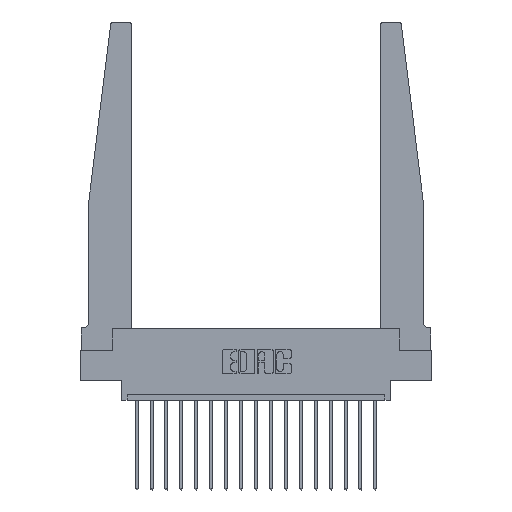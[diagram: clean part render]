
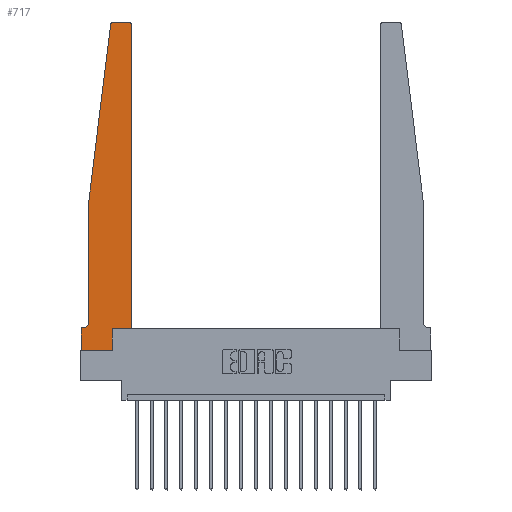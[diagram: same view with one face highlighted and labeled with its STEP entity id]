
A CAD part, top view. The second image highlights one B-rep face of the part: STEP entity #717.
In plain terms, the highlighted planar face has unit normal (0, 0, 1).
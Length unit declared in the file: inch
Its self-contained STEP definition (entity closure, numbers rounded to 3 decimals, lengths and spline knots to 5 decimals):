
#295 = CARTESIAN_POINT ( 'NONE',  ( 0.425, 0.18, 0.37 ) ) ;
#332 = LINE ( 'NONE', #9347, #19190 ) ;
#488 = DIRECTION ( 'NONE',  ( 1., 0., 0. ) ) ;
#708 = CARTESIAN_POINT ( 'NONE',  ( 0.2605, 0.18, 0.37 ) ) ;
#717 = ADVANCED_FACE ( 'NONE', ( #12326 ), #10765, .T. ) ;
#748 = CARTESIAN_POINT ( 'NONE',  ( 0.395, 2.75, 0.37 ) ) ;
#1298 = VERTEX_POINT ( 'NONE', #6722 ) ;
#1452 = EDGE_CURVE ( 'NONE', #1948, #12382, #332, .T. ) ;
#1479 = ORIENTED_EDGE ( 'NONE', *, *, #14520, .T. ) ;
#1593 = VERTEX_POINT ( 'NONE', #708 ) ;
#1856 = CARTESIAN_POINT ( 'NONE',  ( 0., 0.1875, 0.37 ) ) ;
#1948 = VERTEX_POINT ( 'NONE', #12718 ) ;
#2142 = CARTESIAN_POINT ( 'NONE',  ( 0.27653, 2.72, 0.37 ) ) ;
#3500 = CARTESIAN_POINT ( 'NONE',  ( 0., 0., 0.37 ) ) ;
#3539 = EDGE_CURVE ( 'NONE', #6648, #1298, #10495, .T. ) ;
#4411 = DIRECTION ( 'NONE',  ( -1., 0., 0. ) ) ;
#4610 = AXIS2_PLACEMENT_3D ( 'NONE', #1856, #7816, #14106 ) ;
#4920 = DIRECTION ( 'NONE',  ( 0., 1., 0. ) ) ;
#5121 = VECTOR ( 'NONE', #4411, 39.37008 ) ;
#5451 = VERTEX_POINT ( 'NONE', #6592 ) ;
#5759 = EDGE_CURVE ( 'NONE', #8194, #7303, #10696, .T. ) ;
#5933 = LINE ( 'NONE', #10330, #7290 ) ;
#6024 = VERTEX_POINT ( 'NONE', #8414 ) ;
#6096 = CIRCLE ( 'NONE', #14825, 0.05 ) ;
#6125 = DIRECTION ( 'NONE',  ( 1., 0., 0. ) ) ;
#6316 = CARTESIAN_POINT ( 'NONE',  ( 0.065, 1.25, 0.37 ) ) ;
#6592 = CARTESIAN_POINT ( 'NONE',  ( 0.425, 0.18, 0.37 ) ) ;
#6648 = VERTEX_POINT ( 'NONE', #6976 ) ;
#6722 = CARTESIAN_POINT ( 'NONE',  ( 0.24675, 2.72367, 0.37 ) ) ;
#6766 = DIRECTION ( 'NONE',  ( 0., 0., 1. ) ) ;
#6798 = CARTESIAN_POINT ( 'NONE',  ( 0., 0.1875, 0.37 ) ) ;
#6899 = CARTESIAN_POINT ( 'NONE',  ( 0.065, 0.1875, 0.37 ) ) ;
#6976 = CARTESIAN_POINT ( 'NONE',  ( 0.27653, 2.75, 0.37 ) ) ;
#7077 = ORIENTED_EDGE ( 'NONE', *, *, #9701, .T. ) ;
#7096 = ORIENTED_EDGE ( 'NONE', *, *, #13412, .T. ) ;
#7290 = VECTOR ( 'NONE', #7386, 39.37008 ) ;
#7303 = VERTEX_POINT ( 'NONE', #748 ) ;
#7348 = LINE ( 'NONE', #17659, #5121 ) ;
#7386 = DIRECTION ( 'NONE',  ( 1., 0., 0. ) ) ;
#7409 = ORIENTED_EDGE ( 'NONE', *, *, #5759, .T. ) ;
#7816 = DIRECTION ( 'NONE',  ( 0., 0., 1. ) ) ;
#8069 = DIRECTION ( 'NONE',  ( -0.122, -0.992, 0. ) ) ;
#8194 = VERTEX_POINT ( 'NONE', #18931 ) ;
#8267 = EDGE_CURVE ( 'NONE', #1298, #16769, #15222, .T. ) ;
#8414 = CARTESIAN_POINT ( 'NONE',  ( 0.065, 0.2375, 0.37 ) ) ;
#8739 = ORIENTED_EDGE ( 'NONE', *, *, #10263, .T. ) ;
#8806 = EDGE_CURVE ( 'NONE', #12382, #1593, #18109, .T. ) ;
#8812 = AXIS2_PLACEMENT_3D ( 'NONE', #13911, #6766, #488 ) ;
#8829 = DIRECTION ( 'NONE',  ( -1., 0., 0. ) ) ;
#9012 = VERTEX_POINT ( 'NONE', #12609 ) ;
#9017 = DIRECTION ( 'NONE',  ( 1., 0., 0. ) ) ;
#9347 = CARTESIAN_POINT ( 'NONE',  ( 0., 0., 0.37 ) ) ;
#9701 = EDGE_CURVE ( 'NONE', #1593, #5451, #5933, .T. ) ;
#10263 = EDGE_CURVE ( 'NONE', #5451, #8194, #12343, .T. ) ;
#10330 = CARTESIAN_POINT ( 'NONE',  ( 0.425, 0.18, 0.37 ) ) ;
#10352 = VECTOR ( 'NONE', #12438, 39.37008 ) ;
#10495 = CIRCLE ( 'NONE', #12678, 0.03 ) ;
#10648 = EDGE_CURVE ( 'NONE', #16696, #1948, #12778, .T. ) ;
#10696 = CIRCLE ( 'NONE', #8812, 0.03 ) ;
#10765 = PLANE ( 'NONE',  #4610 ) ;
#10926 = ORIENTED_EDGE ( 'NONE', *, *, #1452, .T. ) ;
#11382 = VECTOR ( 'NONE', #12855, 39.37008 ) ;
#11777 = VECTOR ( 'NONE', #18991, 39.37008 ) ;
#11908 = ORIENTED_EDGE ( 'NONE', *, *, #3539, .T. ) ;
#12326 = FACE_OUTER_BOUND ( 'NONE', #18128, .T. ) ;
#12343 = LINE ( 'NONE', #295, #14545 ) ;
#12382 = VERTEX_POINT ( 'NONE', #18902 ) ;
#12438 = DIRECTION ( 'NONE',  ( 0., 1., 0. ) ) ;
#12487 = ORIENTED_EDGE ( 'NONE', *, *, #17107, .T. ) ;
#12516 = DIRECTION ( 'NONE',  ( 0., 0., 1. ) ) ;
#12609 = CARTESIAN_POINT ( 'NONE',  ( 0.015, 0.1875, 0.37 ) ) ;
#12678 = AXIS2_PLACEMENT_3D ( 'NONE', #2142, #12516, #9017 ) ;
#12718 = CARTESIAN_POINT ( 'NONE',  ( 0., 0., 0.37 ) ) ;
#12778 = LINE ( 'NONE', #3500, #18246 ) ;
#12855 = DIRECTION ( 'NONE',  ( -1., 0., 0. ) ) ;
#13101 = CARTESIAN_POINT ( 'NONE',  ( 0.065, 1.25, 0.37 ) ) ;
#13412 = EDGE_CURVE ( 'NONE', #7303, #6648, #7348, .T. ) ;
#13439 = DIRECTION ( 'NONE',  ( 0., 0., -1. ) ) ;
#13595 = CARTESIAN_POINT ( 'NONE',  ( 0.2605, 0.18, 0.37 ) ) ;
#13778 = ORIENTED_EDGE ( 'NONE', *, *, #8806, .T. ) ;
#13911 = CARTESIAN_POINT ( 'NONE',  ( 0.395, 2.72, 0.37 ) ) ;
#14106 = DIRECTION ( 'NONE',  ( 1., 0., 0. ) ) ;
#14260 = DIRECTION ( 'NONE',  ( 0., -1., 0. ) ) ;
#14413 = VECTOR ( 'NONE', #8069, 39.37008 ) ;
#14520 = EDGE_CURVE ( 'NONE', #9012, #16696, #17104, .T. ) ;
#14545 = VECTOR ( 'NONE', #4920, 39.37008 ) ;
#14825 = AXIS2_PLACEMENT_3D ( 'NONE', #16323, #13439, #8829 ) ;
#15222 = LINE ( 'NONE', #6316, #14413 ) ;
#15655 = ORIENTED_EDGE ( 'NONE', *, *, #10648, .T. ) ;
#16323 = CARTESIAN_POINT ( 'NONE',  ( 0.015, 0.2375, 0.37 ) ) ;
#16696 = VERTEX_POINT ( 'NONE', #6798 ) ;
#16769 = VERTEX_POINT ( 'NONE', #16909 ) ;
#16909 = CARTESIAN_POINT ( 'NONE',  ( 0.065, 1.25, 0.37 ) ) ;
#17104 = LINE ( 'NONE', #6899, #11382 ) ;
#17107 = EDGE_CURVE ( 'NONE', #6024, #9012, #6096, .T. ) ;
#17659 = CARTESIAN_POINT ( 'NONE',  ( 0.25, 2.75, 0.37 ) ) ;
#17843 = ORIENTED_EDGE ( 'NONE', *, *, #8267, .T. ) ;
#18109 = LINE ( 'NONE', #13595, #10352 ) ;
#18128 = EDGE_LOOP ( 'NONE', ( #7096, #11908, #17843, #19223, #12487, #1479, #15655, #10926, #13778, #7077, #8739, #7409 ) ) ;
#18246 = VECTOR ( 'NONE', #14260, 39.37008 ) ;
#18897 = LINE ( 'NONE', #13101, #11777 ) ;
#18902 = CARTESIAN_POINT ( 'NONE',  ( 0.2605, 0., 0.37 ) ) ;
#18931 = CARTESIAN_POINT ( 'NONE',  ( 0.425, 2.72, 0.37 ) ) ;
#18991 = DIRECTION ( 'NONE',  ( 0., -1., 0. ) ) ;
#19149 = EDGE_CURVE ( 'NONE', #16769, #6024, #18897, .T. ) ;
#19190 = VECTOR ( 'NONE', #6125, 39.37008 ) ;
#19223 = ORIENTED_EDGE ( 'NONE', *, *, #19149, .T. ) ;
